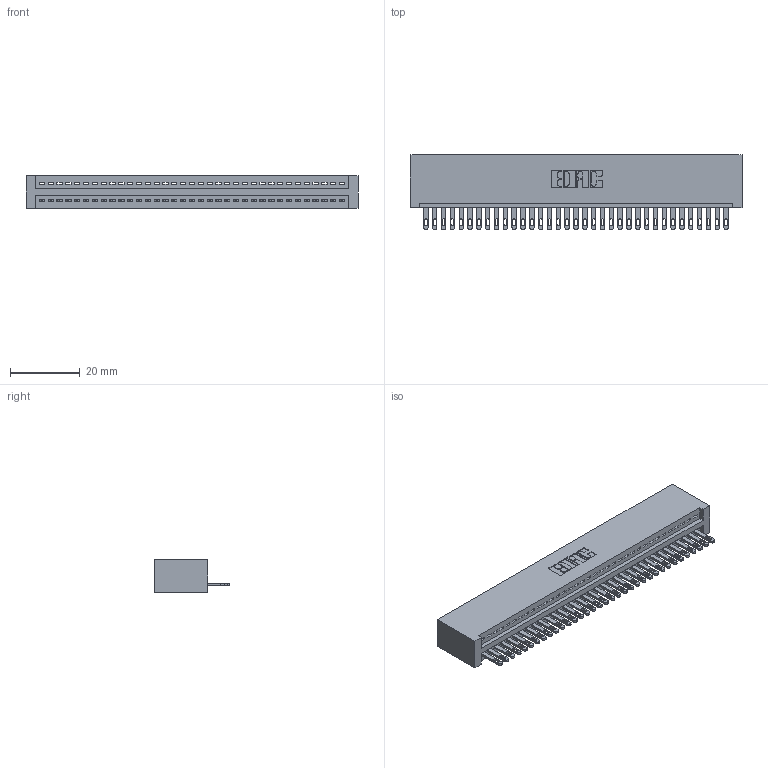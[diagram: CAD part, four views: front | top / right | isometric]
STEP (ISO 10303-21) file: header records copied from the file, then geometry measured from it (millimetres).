
FILE_DESCRIPTION (( 'STEP AP203' ), '1' );
FILE_NAME ('345-035-500-101.STEP', '2019-10-07T20:02:07', ( '' ), ( '' ), 'SwSTEP 2.0', 'SolidWorks 2016', '' );
FILE_SCHEMA (( 'CONFIG_CONTROL_DESIGN' ));
Length unit declared in the file: inch
Products named in the file (3): 345-035-500-101; 345-292-001_345-293-100; 345 Part_No Mounting Lugs
Assembly tree (36 placements, depth 2):
  345-035-500-101
    345 Part_No Mounting Lugs
    345-292-001_345-293-100  x35
Bounding box: 95.5 x 21.51 x 9.4 mm (x, y, z)
Volume: 9619.7 mm3; surface area: 12957.4 mm2
Topology: 36 solids, 36 shells, 2008 faces, 6197 edges, 4130 vertices
Faces by surface type: plane 1266, cylinder 742
Entity records: 26937 total; most frequent: CARTESIAN_POINT 4673, ORIENTED_EDGE 4642, DIRECTION 4087, EDGE_CURVE 2321, LINE 2053, VECTOR 2053, VERTEX_POINT 1546, AXIS2_PLACEMENT_3D 1017
